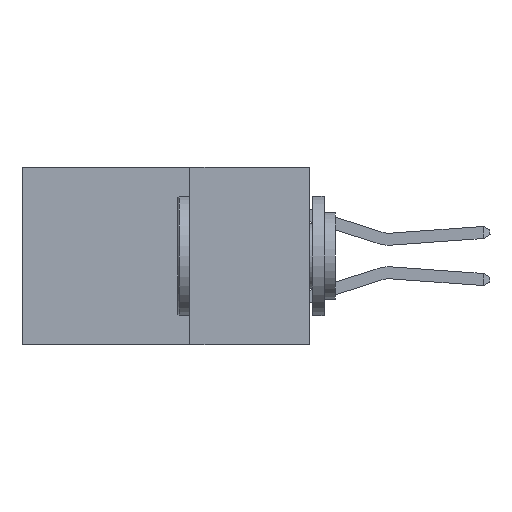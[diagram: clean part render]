
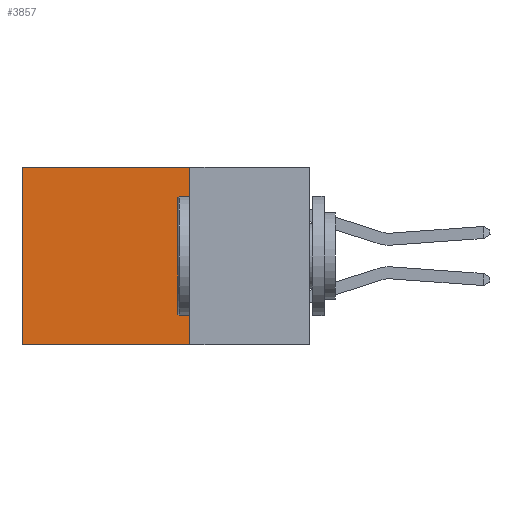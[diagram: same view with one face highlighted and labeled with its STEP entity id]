
A CAD part, left-side view. The second image highlights one B-rep face of the part: STEP entity #3857.
In plain terms, the highlighted planar face has unit normal (-1, 0, 0).
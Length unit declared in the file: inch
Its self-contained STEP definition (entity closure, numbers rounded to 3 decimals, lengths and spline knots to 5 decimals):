
#582 = LINE ( 'NONE', #6896, #13184 ) ;
#650 = CARTESIAN_POINT ( 'NONE',  ( 0.298, 0.25, 0. ) ) ;
#655 = PLANE ( 'NONE',  #3000 ) ;
#3000 = AXIS2_PLACEMENT_3D ( 'NONE', #20792, #20676, #5580 ) ;
#3413 = VECTOR ( 'NONE', #5349, 39.37008 ) ;
#3857 = ADVANCED_FACE ( 'NONE', ( #3912 ), #655, .F. ) ;
#3912 = FACE_OUTER_BOUND ( 'NONE', #30053, .T. ) ;
#5068 = VERTEX_POINT ( 'NONE', #30432 ) ;
#5349 = DIRECTION ( 'NONE',  ( 0., 1., 0. ) ) ;
#5580 = DIRECTION ( 'NONE',  ( 0., 0., -1. ) ) ;
#6896 = CARTESIAN_POINT ( 'NONE',  ( 0.298, 0.25, -0.37 ) ) ;
#6974 = CARTESIAN_POINT ( 'NONE',  ( 0.298, 0.6, -0.37 ) ) ;
#7838 = CARTESIAN_POINT ( 'NONE',  ( 0.298, 0.25, 0. ) ) ;
#9596 = VERTEX_POINT ( 'NONE', #6974 ) ;
#10394 = DIRECTION ( 'NONE',  ( 0., 0., -1. ) ) ;
#10787 = VECTOR ( 'NONE', #10394, 39.37008 ) ;
#13184 = VECTOR ( 'NONE', #29882, 39.37008 ) ;
#13884 = CARTESIAN_POINT ( 'NONE',  ( 0.298, 0.25, -0.37 ) ) ;
#14104 = EDGE_CURVE ( 'NONE', #5068, #9596, #30528, .T. ) ;
#14120 = VERTEX_POINT ( 'NONE', #7838 ) ;
#14488 = EDGE_CURVE ( 'NONE', #31659, #9596, #582, .T. ) ;
#14542 = CARTESIAN_POINT ( 'NONE',  ( 0.298, 0.25, 0. ) ) ;
#15005 = ORIENTED_EDGE ( 'NONE', *, *, #14488, .F. ) ;
#16972 = EDGE_CURVE ( 'NONE', #14120, #31659, #28746, .T. ) ;
#20135 = EDGE_CURVE ( 'NONE', #14120, #5068, #30250, .T. ) ;
#20676 = DIRECTION ( 'NONE',  ( 1., 0., 0. ) ) ;
#20792 = CARTESIAN_POINT ( 'NONE',  ( 0.298, 0.25, 0. ) ) ;
#22844 = ORIENTED_EDGE ( 'NONE', *, *, #14104, .T. ) ;
#22957 = CARTESIAN_POINT ( 'NONE',  ( 0.298, 0.6, 0. ) ) ;
#27962 = VECTOR ( 'NONE', #30533, 39.37008 ) ;
#28746 = LINE ( 'NONE', #14542, #27962 ) ;
#29455 = ORIENTED_EDGE ( 'NONE', *, *, #16972, .F. ) ;
#29882 = DIRECTION ( 'NONE',  ( 0., 1., 0. ) ) ;
#30053 = EDGE_LOOP ( 'NONE', ( #22844, #15005, #29455, #30960 ) ) ;
#30250 = LINE ( 'NONE', #650, #3413 ) ;
#30432 = CARTESIAN_POINT ( 'NONE',  ( 0.298, 0.6, 0. ) ) ;
#30528 = LINE ( 'NONE', #22957, #10787 ) ;
#30533 = DIRECTION ( 'NONE',  ( 0., 0., -1. ) ) ;
#30960 = ORIENTED_EDGE ( 'NONE', *, *, #20135, .T. ) ;
#31659 = VERTEX_POINT ( 'NONE', #13884 ) ;
